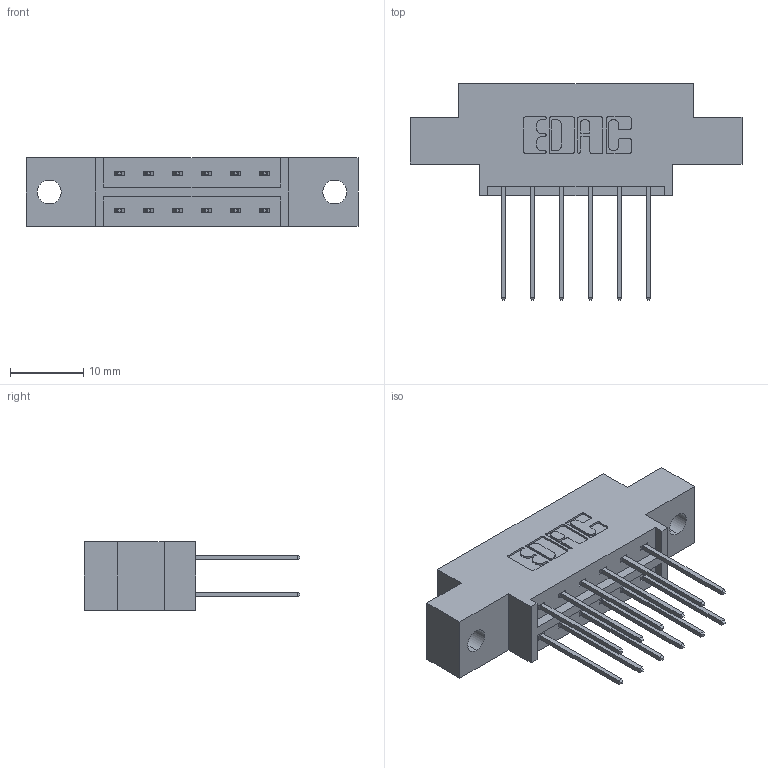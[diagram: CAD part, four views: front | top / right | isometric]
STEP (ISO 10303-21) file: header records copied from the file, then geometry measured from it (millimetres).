
FILE_DESCRIPTION (( 'STEP AP203' ), '1' );
FILE_NAME ('333-012-540-802.STEP', '2018-08-01T00:21:10', ( '' ), ( '' ), 'SwSTEP 2.0', 'SolidWorks 2016', '' );
FILE_SCHEMA (( 'CONFIG_CONTROL_DESIGN' ));
Length unit declared in the file: inch
Products named in the file (3): 333 Part_Offset - .128 Dia; 345-292-001_345-293-140; 333-012-540-802
Assembly tree (13 placements, depth 2):
  333-012-540-802
    333 Part_Offset - .128 Dia
    345-292-001_345-293-140  x12
Bounding box: 45.31 x 29.47 x 9.4 mm (x, y, z)
Volume: 4070.6 mm3; surface area: 4596.5 mm2
Topology: 13 solids, 13 shells, 742 faces, 2183 edges, 1438 vertices
Faces by surface type: plane 506, cylinder 236
Entity records: 8669 total; most frequent: CARTESIAN_POINT 1482, ORIENTED_EDGE 1418, DIRECTION 1329, EDGE_CURVE 709, LINE 581, VECTOR 581, VERTEX_POINT 470, AXIS2_PLACEMENT_3D 374
